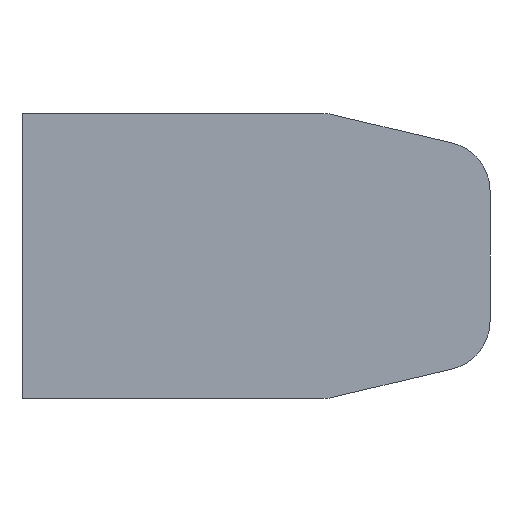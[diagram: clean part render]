
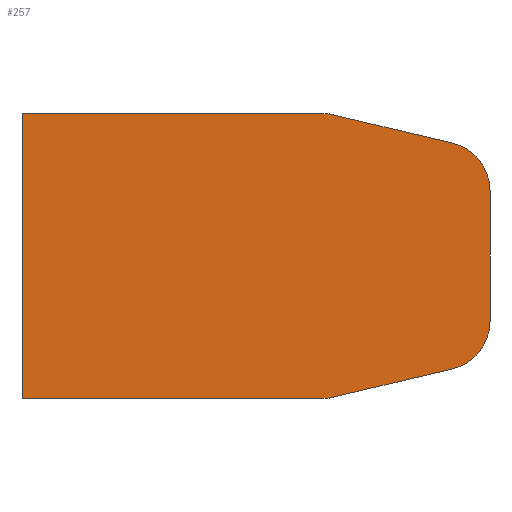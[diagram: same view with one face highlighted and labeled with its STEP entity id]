
A CAD part, front view. The second image highlights one B-rep face of the part: STEP entity #257.
In plain terms, the highlighted planar face has unit normal (0, -1, 0).
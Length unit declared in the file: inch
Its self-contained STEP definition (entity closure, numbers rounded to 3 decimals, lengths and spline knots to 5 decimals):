
#27=PLANE('',#303);
#42=FACE_OUTER_BOUND('',#60,.T.);
#60=EDGE_LOOP('',(#228,#229,#230,#231,#232,#233,#234,#235,#236,#237));
#65=LINE('',#395,#87);
#73=LINE('',#421,#95);
#76=LINE('',#429,#98);
#79=LINE('',#437,#101);
#80=LINE('',#447,#102);
#82=LINE('',#450,#104);
#87=VECTOR('',#318,0.3937);
#95=VECTOR('',#342,0.3937);
#98=VECTOR('',#351,0.3937);
#101=VECTOR('',#360,0.3937);
#102=VECTOR('',#373,0.3937);
#104=VECTOR('',#377,0.3937);
#106=CIRCLE('',#280,0.125);
#111=CIRCLE('',#288,0.125);
#112=CIRCLE('',#291,0.125);
#113=CIRCLE('',#294,0.125);
#118=VERTEX_POINT('',#385);
#119=VERTEX_POINT('',#387);
#121=VERTEX_POINT('',#393);
#130=VERTEX_POINT('',#415);
#131=VERTEX_POINT('',#419);
#132=VERTEX_POINT('',#423);
#133=VERTEX_POINT('',#427);
#134=VERTEX_POINT('',#431);
#135=VERTEX_POINT('',#435);
#138=VERTEX_POINT('',#446);
#141=EDGE_CURVE('',#118,#119,#106,.T.);
#145=EDGE_CURVE('',#121,#118,#65,.T.);
#156=EDGE_CURVE('',#130,#121,#111,.T.);
#158=EDGE_CURVE('',#131,#130,#73,.T.);
#160=EDGE_CURVE('',#132,#131,#112,.T.);
#162=EDGE_CURVE('',#133,#132,#76,.T.);
#164=EDGE_CURVE('',#134,#133,#113,.T.);
#166=EDGE_CURVE('',#135,#134,#79,.T.);
#169=EDGE_CURVE('',#138,#135,#80,.T.);
#171=EDGE_CURVE('',#119,#138,#82,.T.);
#228=ORIENTED_EDGE('',*,*,#141,.F.);
#229=ORIENTED_EDGE('',*,*,#145,.F.);
#230=ORIENTED_EDGE('',*,*,#156,.F.);
#231=ORIENTED_EDGE('',*,*,#158,.F.);
#232=ORIENTED_EDGE('',*,*,#160,.F.);
#233=ORIENTED_EDGE('',*,*,#162,.F.);
#234=ORIENTED_EDGE('',*,*,#164,.F.);
#235=ORIENTED_EDGE('',*,*,#166,.F.);
#236=ORIENTED_EDGE('',*,*,#169,.F.);
#237=ORIENTED_EDGE('',*,*,#171,.F.);
#257=ADVANCED_FACE('',(#42),#27,.F.);
#280=AXIS2_PLACEMENT_3D('',#388,#311,#312);
#288=AXIS2_PLACEMENT_3D('',#417,#337,#338);
#291=AXIS2_PLACEMENT_3D('',#425,#346,#347);
#294=AXIS2_PLACEMENT_3D('',#433,#355,#356);
#303=AXIS2_PLACEMENT_3D('',#451,#378,#379);
#311=DIRECTION('center_axis',(0.,1.,0.));
#312=DIRECTION('ref_axis',(0.116,0.,-0.993));
#318=DIRECTION('',(-0.973,0.,-0.231));
#337=DIRECTION('center_axis',(0.,1.,0.));
#338=DIRECTION('ref_axis',(0.785,0.,-0.62));
#342=DIRECTION('',(0.,0.,-1.));
#346=DIRECTION('center_axis',(0.,1.,0.));
#347=DIRECTION('ref_axis',(0.785,0.,0.62));
#351=DIRECTION('',(0.973,0.,-0.231));
#355=DIRECTION('center_axis',(0.,1.,0.));
#356=DIRECTION('ref_axis',(0.116,0.,0.993));
#360=DIRECTION('',(1.,0.,0.));
#373=DIRECTION('',(0.,0.,1.));
#377=DIRECTION('',(-1.,0.,0.));
#378=DIRECTION('center_axis',(0.,1.,0.));
#379=DIRECTION('ref_axis',(0.,0.,1.));
#385=CARTESIAN_POINT('',(0.79224,0.,-0.72362));
#387=CARTESIAN_POINT('',(0.76337,0.,-0.727));
#388=CARTESIAN_POINT('Origin',(0.76337,0.,-0.602));
#393=CARTESIAN_POINT('',(1.09687,0.,-0.65132));
#395=CARTESIAN_POINT('',(1.193,0.,-0.6285));
#415=CARTESIAN_POINT('',(1.193,0.,-0.5297));
#417=CARTESIAN_POINT('Origin',(1.068,0.,-0.5297));
#419=CARTESIAN_POINT('',(1.193,0.,-0.1973));
#421=CARTESIAN_POINT('',(1.193,0.,-0.0985));
#423=CARTESIAN_POINT('',(1.09687,0.,-0.07568));
#425=CARTESIAN_POINT('Origin',(1.068,0.,-0.1973));
#427=CARTESIAN_POINT('',(0.79224,0.,-0.00338));
#429=CARTESIAN_POINT('',(0.778,0.,0.));
#431=CARTESIAN_POINT('',(0.76337,0.,0.));
#433=CARTESIAN_POINT('Origin',(0.76337,0.,-0.125));
#435=CARTESIAN_POINT('',(0.,0.,0.));
#437=CARTESIAN_POINT('',(0.,0.,0.));
#446=CARTESIAN_POINT('',(0.,0.,-0.727));
#447=CARTESIAN_POINT('',(0.,0.,-0.727));
#450=CARTESIAN_POINT('',(0.778,0.,-0.727));
#451=CARTESIAN_POINT('Origin',(0.56689,0.,-0.3635));
